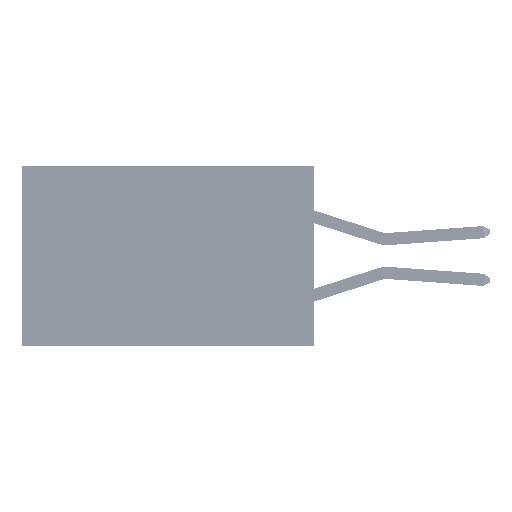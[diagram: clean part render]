
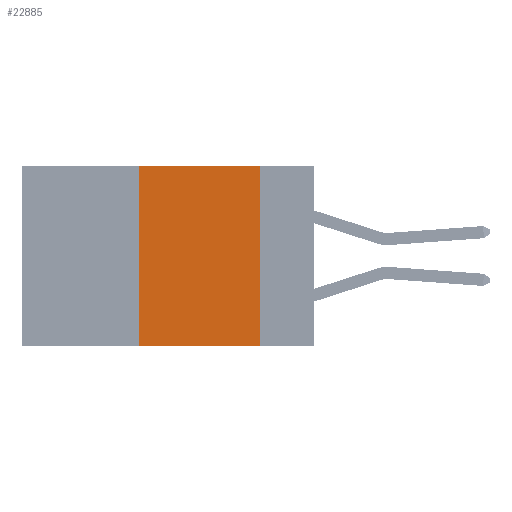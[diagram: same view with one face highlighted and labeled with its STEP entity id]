
A CAD part, left-side view. The second image highlights one B-rep face of the part: STEP entity #22885.
In plain terms, the highlighted planar face has unit normal (-1, 0, 0).
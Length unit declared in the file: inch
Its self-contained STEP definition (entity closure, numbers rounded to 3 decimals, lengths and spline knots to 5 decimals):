
#3136 = LINE ( 'NONE', #24733, #14406 ) ;
#3298 = EDGE_LOOP ( 'NONE', ( #8443, #18669, #37572, #9589 ) ) ;
#3586 = EDGE_CURVE ( 'NONE', #20392, #46170, #3136, .T. ) ;
#5569 = DIRECTION ( 'NONE',  ( 0., -1., 0. ) ) ;
#5714 = CARTESIAN_POINT ( 'NONE',  ( 0., 0.6, 0. ) ) ;
#8338 = CARTESIAN_POINT ( 'NONE',  ( 0., 0.11, 0. ) ) ;
#8443 = ORIENTED_EDGE ( 'NONE', *, *, #9473, .F. ) ;
#9473 = EDGE_CURVE ( 'NONE', #34932, #46170, #42449, .T. ) ;
#9589 = ORIENTED_EDGE ( 'NONE', *, *, #3586, .T. ) ;
#10318 = DIRECTION ( 'NONE',  ( 0., -1., 0. ) ) ;
#10445 = CARTESIAN_POINT ( 'NONE',  ( 0., 0.36, -0.37 ) ) ;
#14406 = VECTOR ( 'NONE', #10318, 39.37008 ) ;
#15603 = LINE ( 'NONE', #25531, #38148 ) ;
#15726 = DIRECTION ( 'NONE',  ( 1., 0., 0. ) ) ;
#16128 = CARTESIAN_POINT ( 'NONE',  ( 0., 0.11, 0. ) ) ;
#18454 = AXIS2_PLACEMENT_3D ( 'NONE', #33273, #15726, #44468 ) ;
#18669 = ORIENTED_EDGE ( 'NONE', *, *, #45233, .F. ) ;
#20392 = VERTEX_POINT ( 'NONE', #10445 ) ;
#21331 = VECTOR ( 'NONE', #5569, 39.37008 ) ;
#22885 = ADVANCED_FACE ( 'NONE', ( #40619 ), #32977, .F. ) ;
#24733 = CARTESIAN_POINT ( 'NONE',  ( 0., 0.6, -0.37 ) ) ;
#25531 = CARTESIAN_POINT ( 'NONE',  ( 0., 0.36, 0. ) ) ;
#27586 = LINE ( 'NONE', #5714, #21331 ) ;
#32977 = PLANE ( 'NONE',  #18454 ) ;
#33273 = CARTESIAN_POINT ( 'NONE',  ( 0., 0.6, 0. ) ) ;
#34932 = VERTEX_POINT ( 'NONE', #8338 ) ;
#36216 = VECTOR ( 'NONE', #41393, 39.37008 ) ;
#37572 = ORIENTED_EDGE ( 'NONE', *, *, #39976, .F. ) ;
#37790 = CARTESIAN_POINT ( 'NONE',  ( 0., 0.11, -0.37 ) ) ;
#38148 = VECTOR ( 'NONE', #40953, 39.37008 ) ;
#39976 = EDGE_CURVE ( 'NONE', #20392, #40173, #15603, .T. ) ;
#40173 = VERTEX_POINT ( 'NONE', #41572 ) ;
#40619 = FACE_OUTER_BOUND ( 'NONE', #3298, .T. ) ;
#40953 = DIRECTION ( 'NONE',  ( 0., 0., 1. ) ) ;
#41393 = DIRECTION ( 'NONE',  ( 0., 0., -1. ) ) ;
#41572 = CARTESIAN_POINT ( 'NONE',  ( 0., 0.36, 0. ) ) ;
#42449 = LINE ( 'NONE', #16128, #36216 ) ;
#44468 = DIRECTION ( 'NONE',  ( 0., 0., -1. ) ) ;
#45233 = EDGE_CURVE ( 'NONE', #40173, #34932, #27586, .T. ) ;
#46170 = VERTEX_POINT ( 'NONE', #37790 ) ;
